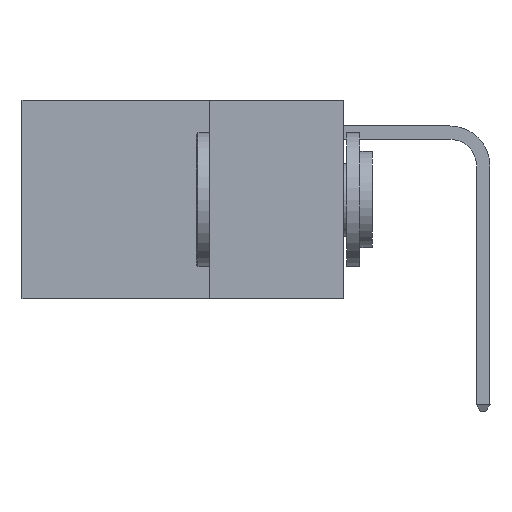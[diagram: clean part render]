
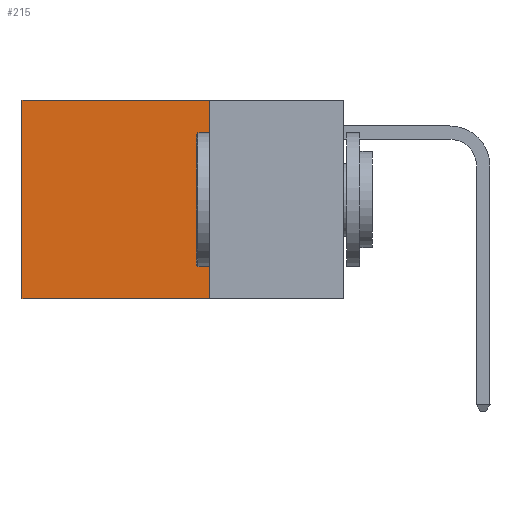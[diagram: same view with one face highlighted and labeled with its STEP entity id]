
A CAD part, left-side view. The second image highlights one B-rep face of the part: STEP entity #215.
In plain terms, the highlighted planar face has unit normal (-1, 0, 0).
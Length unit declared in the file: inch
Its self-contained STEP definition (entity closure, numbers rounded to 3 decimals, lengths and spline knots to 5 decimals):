
#57 = AXIS2_PLACEMENT_3D ( 'NONE', #1741, #1036, #893 ) ;
#124 = DIRECTION ( 'NONE',  ( 0., 0., -1. ) ) ;
#186 = EDGE_CURVE ( 'NONE', #10327, #8029, #1884, .T. ) ;
#215 = ADVANCED_FACE ( 'NONE', ( #1768 ), #2033, .F. ) ;
#372 = EDGE_CURVE ( 'NONE', #2026, #11992, #1329, .T. ) ;
#893 = DIRECTION ( 'NONE',  ( 0., 0., -1. ) ) ;
#1036 = DIRECTION ( 'NONE',  ( 1., 0., 0. ) ) ;
#1068 = CARTESIAN_POINT ( 'NONE',  ( 0.2625, 0.25, 0. ) ) ;
#1279 = VECTOR ( 'NONE', #124, 39.37008 ) ;
#1304 = ORIENTED_EDGE ( 'NONE', *, *, #10681, .F. ) ;
#1329 = LINE ( 'NONE', #11318, #1279 ) ;
#1741 = CARTESIAN_POINT ( 'NONE',  ( 0.2625, 0.25, 0. ) ) ;
#1768 = FACE_OUTER_BOUND ( 'NONE', #4904, .T. ) ;
#1834 = VECTOR ( 'NONE', #4320, 39.37008 ) ;
#1884 = LINE ( 'NONE', #5440, #1834 ) ;
#1887 = CARTESIAN_POINT ( 'NONE',  ( 0.2625, 0.25, -0.37 ) ) ;
#1896 = LINE ( 'NONE', #2712, #9621 ) ;
#2026 = VERTEX_POINT ( 'NONE', #7608 ) ;
#2033 = PLANE ( 'NONE',  #57 ) ;
#2712 = CARTESIAN_POINT ( 'NONE',  ( 0.2625, 0.25, -0.37 ) ) ;
#4320 = DIRECTION ( 'NONE',  ( 0., 0., -1. ) ) ;
#4904 = EDGE_LOOP ( 'NONE', ( #11115, #1304, #9256, #10728 ) ) ;
#5440 = CARTESIAN_POINT ( 'NONE',  ( 0.2625, 0.25, 0. ) ) ;
#7480 = CARTESIAN_POINT ( 'NONE',  ( 0.2625, 0.25, 0. ) ) ;
#7608 = CARTESIAN_POINT ( 'NONE',  ( 0.2625, 0.6, 0. ) ) ;
#8029 = VERTEX_POINT ( 'NONE', #1887 ) ;
#8715 = DIRECTION ( 'NONE',  ( 0., 1., 0. ) ) ;
#9256 = ORIENTED_EDGE ( 'NONE', *, *, #186, .F. ) ;
#9621 = VECTOR ( 'NONE', #8715, 39.37008 ) ;
#9807 = CARTESIAN_POINT ( 'NONE',  ( 0.2625, 0.6, -0.37 ) ) ;
#10327 = VERTEX_POINT ( 'NONE', #1068 ) ;
#10681 = EDGE_CURVE ( 'NONE', #8029, #11992, #1896, .T. ) ;
#10728 = ORIENTED_EDGE ( 'NONE', *, *, #11203, .T. ) ;
#11115 = ORIENTED_EDGE ( 'NONE', *, *, #372, .T. ) ;
#11203 = EDGE_CURVE ( 'NONE', #10327, #2026, #12855, .T. ) ;
#11318 = CARTESIAN_POINT ( 'NONE',  ( 0.2625, 0.6, 0. ) ) ;
#11431 = DIRECTION ( 'NONE',  ( 0., 1., 0. ) ) ;
#11992 = VERTEX_POINT ( 'NONE', #9807 ) ;
#12572 = VECTOR ( 'NONE', #11431, 39.37008 ) ;
#12855 = LINE ( 'NONE', #7480, #12572 ) ;
